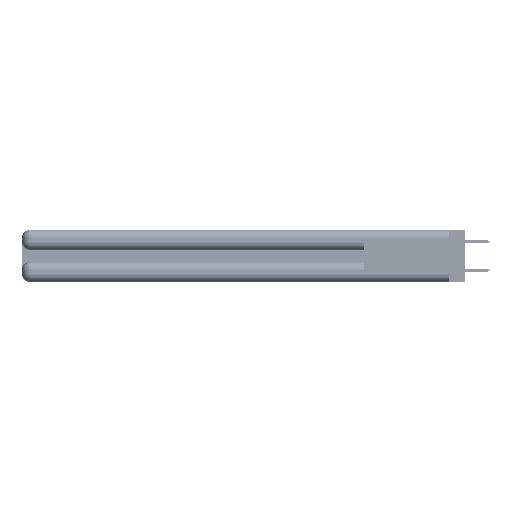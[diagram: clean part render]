
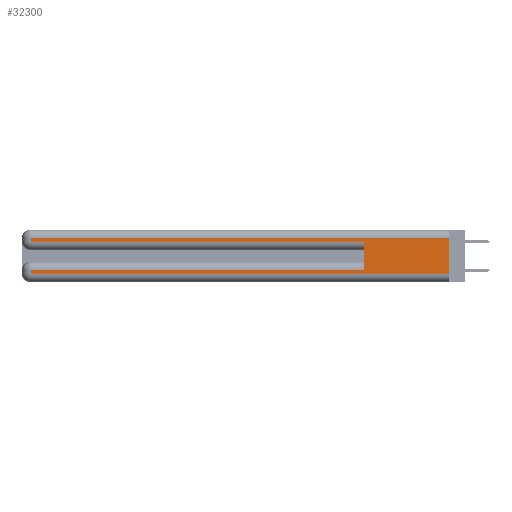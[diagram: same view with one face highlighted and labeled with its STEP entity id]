
A CAD part, left-side view. The second image highlights one B-rep face of the part: STEP entity #32300.
In plain terms, the highlighted planar face has unit normal (-1, 0, 0).
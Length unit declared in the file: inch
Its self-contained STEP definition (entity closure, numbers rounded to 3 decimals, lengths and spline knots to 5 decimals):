
#1112 = VERTEX_POINT ( 'NONE', #29459 ) ;
#3195 = LINE ( 'NONE', #19093, #48939 ) ;
#3565 = LINE ( 'NONE', #51278, #22855 ) ;
#6972 = EDGE_CURVE ( 'NONE', #1112, #25015, #12334, .T. ) ;
#8243 = EDGE_CURVE ( 'NONE', #41813, #36683, #39931, .T. ) ;
#9104 = DIRECTION ( 'NONE',  ( 0., -1., 0. ) ) ;
#10540 = EDGE_CURVE ( 'NONE', #28023, #12583, #33812, .T. ) ;
#10547 = EDGE_CURVE ( 'NONE', #40843, #51259, #3565, .T. ) ;
#11164 = DIRECTION ( 'NONE',  ( 0., 1., 0. ) ) ;
#11418 = ORIENTED_EDGE ( 'NONE', *, *, #40024, .T. ) ;
#12276 = LINE ( 'NONE', #25487, #48371 ) ;
#12334 = LINE ( 'NONE', #31150, #32949 ) ;
#12583 = VERTEX_POINT ( 'NONE', #32144 ) ;
#13485 = CARTESIAN_POINT ( 'NONE',  ( 0., 2.94, 0.06 ) ) ;
#14843 = CARTESIAN_POINT ( 'NONE',  ( 0., 0.6, 0.145 ) ) ;
#15118 = DIRECTION ( 'NONE',  ( 0., 0., -1. ) ) ;
#19093 = CARTESIAN_POINT ( 'NONE',  ( 0., 0., 0.085 ) ) ;
#20710 = AXIS2_PLACEMENT_3D ( 'NONE', #21184, #25299, #50356 ) ;
#20858 = CARTESIAN_POINT ( 'NONE',  ( 0., 2.94, 0.285 ) ) ;
#20923 = VECTOR ( 'NONE', #38040, 39.37008 ) ;
#20931 = FACE_OUTER_BOUND ( 'NONE', #53331, .T. ) ;
#21184 = CARTESIAN_POINT ( 'NONE',  ( 0., 0., 0.37 ) ) ;
#22855 = VECTOR ( 'NONE', #39218, 39.37008 ) ;
#23630 = ORIENTED_EDGE ( 'NONE', *, *, #36375, .T. ) ;
#23888 = EDGE_CURVE ( 'NONE', #1112, #41813, #31867, .T. ) ;
#24606 = CARTESIAN_POINT ( 'NONE',  ( 0., 0., 0.06 ) ) ;
#25015 = VERTEX_POINT ( 'NONE', #42078 ) ;
#25051 = VECTOR ( 'NONE', #40571, 39.37008 ) ;
#25299 = DIRECTION ( 'NONE',  ( 1., 0., 0. ) ) ;
#25487 = CARTESIAN_POINT ( 'NONE',  ( 0., 0., 0.285 ) ) ;
#26504 = ORIENTED_EDGE ( 'NONE', *, *, #10540, .F. ) ;
#26732 = EDGE_CURVE ( 'NONE', #51259, #25015, #41778, .T. ) ;
#26938 = DIRECTION ( 'NONE',  ( 0., 0., 1. ) ) ;
#28023 = VERTEX_POINT ( 'NONE', #32416 ) ;
#28100 = CARTESIAN_POINT ( 'NONE',  ( 0., 2.94, 0.37 ) ) ;
#29010 = CARTESIAN_POINT ( 'NONE',  ( 0., 2.94, 0.31 ) ) ;
#29459 = CARTESIAN_POINT ( 'NONE',  ( 0., 0., 0.31 ) ) ;
#29991 = PLANE ( 'NONE',  #20710 ) ;
#30429 = CARTESIAN_POINT ( 'NONE',  ( 0., 0., 0.31 ) ) ;
#31023 = ORIENTED_EDGE ( 'NONE', *, *, #26732, .T. ) ;
#31150 = CARTESIAN_POINT ( 'NONE',  ( 0., 0., 0.37 ) ) ;
#31526 = ORIENTED_EDGE ( 'NONE', *, *, #6972, .F. ) ;
#31867 = LINE ( 'NONE', #30429, #20923 ) ;
#32067 = VECTOR ( 'NONE', #48952, 39.37008 ) ;
#32144 = CARTESIAN_POINT ( 'NONE',  ( 0., 0.6, 0.285 ) ) ;
#32300 = ADVANCED_FACE ( 'NONE', ( #20931 ), #29991, .F. ) ;
#32347 = ORIENTED_EDGE ( 'NONE', *, *, #23888, .T. ) ;
#32416 = CARTESIAN_POINT ( 'NONE',  ( 0., 0.6, 0.085 ) ) ;
#32949 = VECTOR ( 'NONE', #15118, 39.37008 ) ;
#33812 = LINE ( 'NONE', #14843, #44806 ) ;
#36375 = EDGE_CURVE ( 'NONE', #28023, #40843, #3195, .T. ) ;
#36683 = VERTEX_POINT ( 'NONE', #20858 ) ;
#38040 = DIRECTION ( 'NONE',  ( 0., 1., 0. ) ) ;
#39218 = DIRECTION ( 'NONE',  ( 0., 0., -1. ) ) ;
#39931 = LINE ( 'NONE', #28100, #25051 ) ;
#40024 = EDGE_CURVE ( 'NONE', #36683, #12583, #12276, .T. ) ;
#40571 = DIRECTION ( 'NONE',  ( 0., 0., -1. ) ) ;
#40843 = VERTEX_POINT ( 'NONE', #50481 ) ;
#41778 = LINE ( 'NONE', #24606, #32067 ) ;
#41813 = VERTEX_POINT ( 'NONE', #29010 ) ;
#42078 = CARTESIAN_POINT ( 'NONE',  ( 0., 0., 0.06 ) ) ;
#42279 = ORIENTED_EDGE ( 'NONE', *, *, #8243, .T. ) ;
#44806 = VECTOR ( 'NONE', #26938, 39.37008 ) ;
#44904 = ORIENTED_EDGE ( 'NONE', *, *, #10547, .T. ) ;
#48371 = VECTOR ( 'NONE', #9104, 39.37008 ) ;
#48939 = VECTOR ( 'NONE', #11164, 39.37008 ) ;
#48952 = DIRECTION ( 'NONE',  ( 0., -1., 0. ) ) ;
#50356 = DIRECTION ( 'NONE',  ( 0., 0., -1. ) ) ;
#50481 = CARTESIAN_POINT ( 'NONE',  ( 0., 2.94, 0.085 ) ) ;
#51259 = VERTEX_POINT ( 'NONE', #13485 ) ;
#51278 = CARTESIAN_POINT ( 'NONE',  ( 0., 2.94, 0.37 ) ) ;
#53331 = EDGE_LOOP ( 'NONE', ( #31526, #32347, #42279, #11418, #26504, #23630, #44904, #31023 ) ) ;
